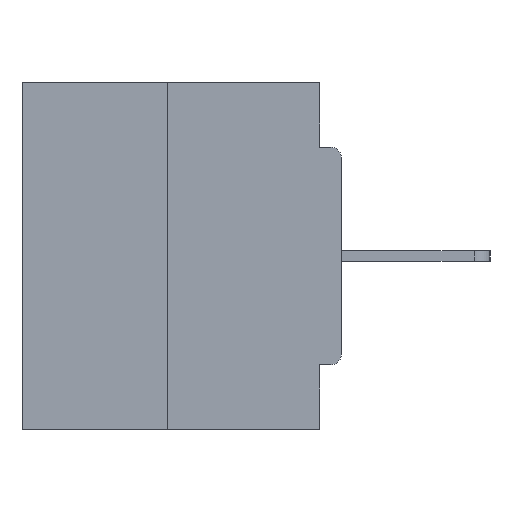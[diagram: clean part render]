
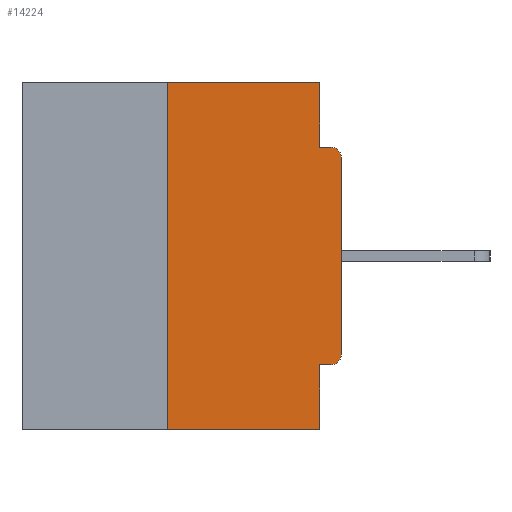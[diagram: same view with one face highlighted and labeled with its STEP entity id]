
A CAD part, left-side view. The second image highlights one B-rep face of the part: STEP entity #14224.
In plain terms, the highlighted planar face has unit normal (-1, 0, 0).
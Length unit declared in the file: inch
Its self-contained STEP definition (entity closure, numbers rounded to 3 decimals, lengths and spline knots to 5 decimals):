
#119 = LINE ( 'NONE', #17995, #26350 ) ;
#186 = ORIENTED_EDGE ( 'NONE', *, *, #22254, .F. ) ;
#590 = EDGE_CURVE ( 'NONE', #14376, #13963, #32036, .T. ) ;
#3729 = DIRECTION ( 'NONE',  ( 0., -1., 0. ) ) ;
#3765 = ORIENTED_EDGE ( 'NONE', *, *, #31731, .F. ) ;
#4177 = ORIENTED_EDGE ( 'NONE', *, *, #32691, .F. ) ;
#4306 = CARTESIAN_POINT ( 'NONE',  ( 0., 0.015, -0.1085 ) ) ;
#4398 = EDGE_CURVE ( 'NONE', #15413, #29083, #28302, .T. ) ;
#4578 = ORIENTED_EDGE ( 'NONE', *, *, #11278, .F. ) ;
#4655 = CARTESIAN_POINT ( 'NONE',  ( 0., 0.46, 0. ) ) ;
#4716 = LINE ( 'NONE', #24520, #18053 ) ;
#5195 = DIRECTION ( 'NONE',  ( 0., 0., -1. ) ) ;
#5204 = DIRECTION ( 'NONE',  ( -1., 0., 0. ) ) ;
#5860 = CARTESIAN_POINT ( 'NONE',  ( 0., 0.031, -0.5 ) ) ;
#6369 = CARTESIAN_POINT ( 'NONE',  ( 0., 0.031, -0.4065 ) ) ;
#6718 = CARTESIAN_POINT ( 'NONE',  ( 0., 0.031, 0. ) ) ;
#6828 = CARTESIAN_POINT ( 'NONE',  ( 0., 0.25, -0.5 ) ) ;
#7240 = DIRECTION ( 'NONE',  ( 0., 0., -1. ) ) ;
#7302 = VERTEX_POINT ( 'NONE', #6369 ) ;
#7743 = DIRECTION ( 'NONE',  ( 0., -1., 0. ) ) ;
#8078 = VECTOR ( 'NONE', #9310, 39.37008 ) ;
#8185 = DIRECTION ( 'NONE',  ( -1., 0., 0. ) ) ;
#8507 = LINE ( 'NONE', #16922, #21374 ) ;
#8883 = LINE ( 'NONE', #6718, #8078 ) ;
#9211 = AXIS2_PLACEMENT_3D ( 'NONE', #23455, #8185, #25909 ) ;
#9310 = DIRECTION ( 'NONE',  ( 0., 0., -1. ) ) ;
#9426 = ORIENTED_EDGE ( 'NONE', *, *, #590, .T. ) ;
#10178 = FACE_OUTER_BOUND ( 'NONE', #28148, .T. ) ;
#11278 = EDGE_CURVE ( 'NONE', #15413, #25139, #17718, .T. ) ;
#11320 = VECTOR ( 'NONE', #28894, 39.37008 ) ;
#12055 = CARTESIAN_POINT ( 'NONE',  ( 0., 0.25, 0. ) ) ;
#12126 = AXIS2_PLACEMENT_3D ( 'NONE', #4655, #22563, #7240 ) ;
#13064 = EDGE_CURVE ( 'NONE', #27603, #14376, #4716, .T. ) ;
#13106 = AXIS2_PLACEMENT_3D ( 'NONE', #4306, #5204, #5195 ) ;
#13963 = VERTEX_POINT ( 'NONE', #30714 ) ;
#14224 = ADVANCED_FACE ( 'NONE', ( #10178 ), #20030, .F. ) ;
#14376 = VERTEX_POINT ( 'NONE', #28000 ) ;
#14650 = ORIENTED_EDGE ( 'NONE', *, *, #19507, .T. ) ;
#15396 = EDGE_CURVE ( 'NONE', #16770, #22059, #8883, .T. ) ;
#15413 = VERTEX_POINT ( 'NONE', #6828 ) ;
#16645 = CARTESIAN_POINT ( 'NONE',  ( 0., 0.46, -0.5 ) ) ;
#16770 = VERTEX_POINT ( 'NONE', #25283 ) ;
#16922 = CARTESIAN_POINT ( 'NONE',  ( 0., 0., -0.0935 ) ) ;
#17452 = CARTESIAN_POINT ( 'NONE',  ( 0., 0., -0.3915 ) ) ;
#17718 = LINE ( 'NONE', #29959, #30130 ) ;
#17880 = ORIENTED_EDGE ( 'NONE', *, *, #15396, .F. ) ;
#17901 = CIRCLE ( 'NONE', #9211, 0.015 ) ;
#17995 = CARTESIAN_POINT ( 'NONE',  ( 0., 0.46, 0. ) ) ;
#18053 = VECTOR ( 'NONE', #26973, 39.37008 ) ;
#18675 = DIRECTION ( 'NONE',  ( 0., 0., -1. ) ) ;
#19507 = EDGE_CURVE ( 'NONE', #31931, #27603, #17901, .T. ) ;
#19528 = VECTOR ( 'NONE', #18675, 39.37008 ) ;
#20030 = PLANE ( 'NONE',  #12126 ) ;
#20730 = CARTESIAN_POINT ( 'NONE',  ( 0., 0.031, -0.0935 ) ) ;
#21023 = VECTOR ( 'NONE', #3729, 39.37008 ) ;
#21374 = VECTOR ( 'NONE', #26916, 39.37008 ) ;
#21456 = ORIENTED_EDGE ( 'NONE', *, *, #13064, .T. ) ;
#22059 = VERTEX_POINT ( 'NONE', #20730 ) ;
#22254 = EDGE_CURVE ( 'NONE', #31931, #7302, #24795, .T. ) ;
#22563 = DIRECTION ( 'NONE',  ( 1., 0., 0. ) ) ;
#23455 = CARTESIAN_POINT ( 'NONE',  ( 0., 0.015, -0.3915 ) ) ;
#24520 = CARTESIAN_POINT ( 'NONE',  ( 0., 0., 0. ) ) ;
#24795 = LINE ( 'NONE', #26396, #11320 ) ;
#25139 = VERTEX_POINT ( 'NONE', #12055 ) ;
#25283 = CARTESIAN_POINT ( 'NONE',  ( 0., 0.031, 0. ) ) ;
#25468 = EDGE_CURVE ( 'NONE', #7302, #29083, #32606, .T. ) ;
#25909 = DIRECTION ( 'NONE',  ( 0., 0., -1. ) ) ;
#26350 = VECTOR ( 'NONE', #7743, 39.37008 ) ;
#26396 = CARTESIAN_POINT ( 'NONE',  ( 0., 0., -0.4065 ) ) ;
#26409 = ORIENTED_EDGE ( 'NONE', *, *, #25468, .F. ) ;
#26916 = DIRECTION ( 'NONE',  ( 0., -1., 0. ) ) ;
#26973 = DIRECTION ( 'NONE',  ( 0., 0., 1. ) ) ;
#27603 = VERTEX_POINT ( 'NONE', #17452 ) ;
#28000 = CARTESIAN_POINT ( 'NONE',  ( 0., 0., -0.1085 ) ) ;
#28148 = EDGE_LOOP ( 'NONE', ( #3765, #4578, #31410, #26409, #186, #14650, #21456, #9426, #4177, #17880 ) ) ;
#28302 = LINE ( 'NONE', #16645, #21023 ) ;
#28894 = DIRECTION ( 'NONE',  ( 0., 1., 0. ) ) ;
#29083 = VERTEX_POINT ( 'NONE', #29874 ) ;
#29874 = CARTESIAN_POINT ( 'NONE',  ( 0., 0.031, -0.5 ) ) ;
#29959 = CARTESIAN_POINT ( 'NONE',  ( 0., 0.25, 0. ) ) ;
#30130 = VECTOR ( 'NONE', #32341, 39.37008 ) ;
#30714 = CARTESIAN_POINT ( 'NONE',  ( 0., 0.015, -0.0935 ) ) ;
#31282 = CARTESIAN_POINT ( 'NONE',  ( 0., 0.015, -0.4065 ) ) ;
#31410 = ORIENTED_EDGE ( 'NONE', *, *, #4398, .T. ) ;
#31731 = EDGE_CURVE ( 'NONE', #25139, #16770, #119, .T. ) ;
#31931 = VERTEX_POINT ( 'NONE', #31282 ) ;
#32036 = CIRCLE ( 'NONE', #13106, 0.015 ) ;
#32341 = DIRECTION ( 'NONE',  ( 0., 0., 1. ) ) ;
#32606 = LINE ( 'NONE', #5860, #19528 ) ;
#32691 = EDGE_CURVE ( 'NONE', #22059, #13963, #8507, .T. ) ;
